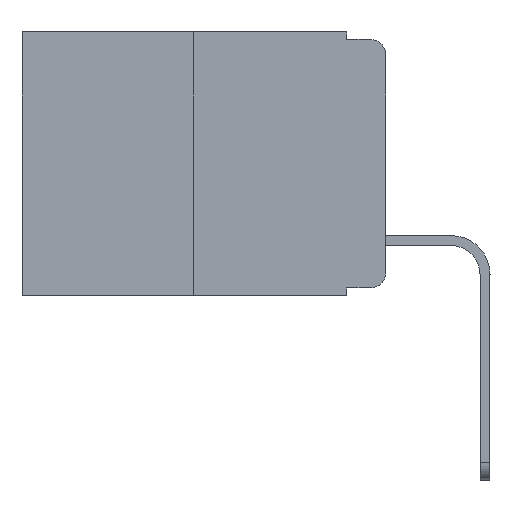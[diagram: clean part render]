
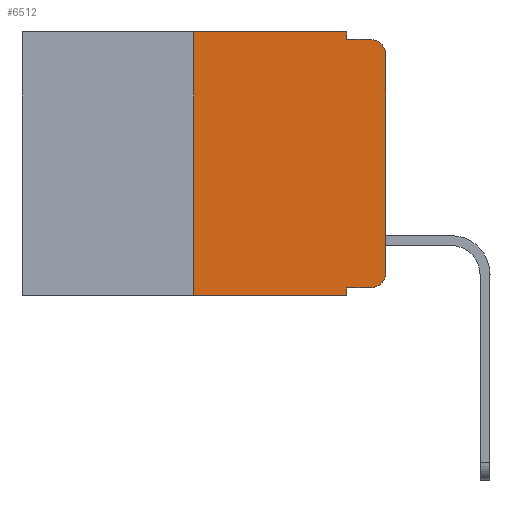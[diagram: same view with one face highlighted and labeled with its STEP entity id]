
A CAD part, left-side view. The second image highlights one B-rep face of the part: STEP entity #6512.
In plain terms, the highlighted planar face has unit normal (-1, 0, 0).
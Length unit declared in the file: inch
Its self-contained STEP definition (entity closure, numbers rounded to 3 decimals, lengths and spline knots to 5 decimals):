
#72 = CARTESIAN_POINT ( 'NONE',  ( 0., 0.051, -0.01 ) ) ;
#123 = CARTESIAN_POINT ( 'NONE',  ( 0., 0.051, 0. ) ) ;
#182 = CARTESIAN_POINT ( 'NONE',  ( 0., 0.25, 0. ) ) ;
#197 = EDGE_CURVE ( 'NONE', #8504, #10785, #8745, .T. ) ;
#387 = LINE ( 'NONE', #72, #3406 ) ;
#425 = VECTOR ( 'NONE', #4775, 39.37008 ) ;
#499 = EDGE_CURVE ( 'NONE', #6750, #7162, #10183, .T. ) ;
#504 = DIRECTION ( 'NONE',  ( 0., 0., -1. ) ) ;
#644 = PLANE ( 'NONE',  #7735 ) ;
#834 = VERTEX_POINT ( 'NONE', #10417 ) ;
#843 = CARTESIAN_POINT ( 'NONE',  ( 0., 0.051, 0. ) ) ;
#847 = ORIENTED_EDGE ( 'NONE', *, *, #5969, .T. ) ;
#1152 = ORIENTED_EDGE ( 'NONE', *, *, #8674, .F. ) ;
#1218 = ORIENTED_EDGE ( 'NONE', *, *, #499, .F. ) ;
#1422 = CARTESIAN_POINT ( 'NONE',  ( 0., 0.473, 0. ) ) ;
#1453 = VERTEX_POINT ( 'NONE', #5334 ) ;
#1470 = DIRECTION ( 'NONE',  ( 0., 0., -1. ) ) ;
#1519 = ORIENTED_EDGE ( 'NONE', *, *, #9599, .T. ) ;
#1961 = VECTOR ( 'NONE', #7259, 39.37008 ) ;
#2309 = DIRECTION ( 'NONE',  ( -1., 0., 0. ) ) ;
#2329 = CARTESIAN_POINT ( 'NONE',  ( 0., 0., -0.313 ) ) ;
#2451 = LINE ( 'NONE', #10314, #9060 ) ;
#2703 = CIRCLE ( 'NONE', #8658, 0.02 ) ;
#2772 = ORIENTED_EDGE ( 'NONE', *, *, #6137, .F. ) ;
#3129 = CARTESIAN_POINT ( 'NONE',  ( 0., 0.02, -0.313 ) ) ;
#3270 = DIRECTION ( 'NONE',  ( 0., 0., -1. ) ) ;
#3406 = VECTOR ( 'NONE', #5617, 39.37008 ) ;
#3453 = VERTEX_POINT ( 'NONE', #2329 ) ;
#3462 = CARTESIAN_POINT ( 'NONE',  ( 0., 0.051, -0.333 ) ) ;
#3577 = CARTESIAN_POINT ( 'NONE',  ( 0., 0.25, 0. ) ) ;
#3778 = EDGE_CURVE ( 'NONE', #834, #1453, #2451, .T. ) ;
#4098 = CARTESIAN_POINT ( 'NONE',  ( 0., 0.02, -0.03 ) ) ;
#4282 = EDGE_LOOP ( 'NONE', ( #847, #1519, #2772, #1152, #1218, #6490, #7884, #6775, #10735, #4455 ) ) ;
#4394 = VERTEX_POINT ( 'NONE', #7450 ) ;
#4455 = ORIENTED_EDGE ( 'NONE', *, *, #5741, .T. ) ;
#4775 = DIRECTION ( 'NONE',  ( 0., -1., 0. ) ) ;
#5334 = CARTESIAN_POINT ( 'NONE',  ( 0., 0.051, -0.343 ) ) ;
#5473 = DIRECTION ( 'NONE',  ( 0., 0., 1. ) ) ;
#5610 = AXIS2_PLACEMENT_3D ( 'NONE', #4098, #2309, #1470 ) ;
#5617 = DIRECTION ( 'NONE',  ( 0., -1., 0. ) ) ;
#5634 = VERTEX_POINT ( 'NONE', #9235 ) ;
#5646 = LINE ( 'NONE', #3577, #9093 ) ;
#5741 = EDGE_CURVE ( 'NONE', #10785, #3453, #2703, .T. ) ;
#5924 = CIRCLE ( 'NONE', #5610, 0.02 ) ;
#5969 = EDGE_CURVE ( 'NONE', #3453, #5634, #7565, .T. ) ;
#6130 = CARTESIAN_POINT ( 'NONE',  ( 0., 0.02, -0.333 ) ) ;
#6137 = EDGE_CURVE ( 'NONE', #4394, #8849, #387, .T. ) ;
#6301 = DIRECTION ( 'NONE',  ( 0., -1., 0. ) ) ;
#6380 = VECTOR ( 'NONE', #11082, 39.37008 ) ;
#6490 = ORIENTED_EDGE ( 'NONE', *, *, #8518, .F. ) ;
#6512 = ADVANCED_FACE ( 'NONE', ( #8415 ), #644, .F. ) ;
#6750 = VERTEX_POINT ( 'NONE', #182 ) ;
#6775 = ORIENTED_EDGE ( 'NONE', *, *, #7632, .F. ) ;
#7162 = VERTEX_POINT ( 'NONE', #843 ) ;
#7188 = DIRECTION ( 'NONE',  ( 0., 0., -1. ) ) ;
#7259 = DIRECTION ( 'NONE',  ( 0., 0., 1. ) ) ;
#7450 = CARTESIAN_POINT ( 'NONE',  ( 0., 0.051, -0.01 ) ) ;
#7565 = LINE ( 'NONE', #9949, #1961 ) ;
#7632 = EDGE_CURVE ( 'NONE', #8504, #1453, #8103, .T. ) ;
#7735 = AXIS2_PLACEMENT_3D ( 'NONE', #1422, #10728, #3270 ) ;
#7884 = ORIENTED_EDGE ( 'NONE', *, *, #3778, .T. ) ;
#7922 = LINE ( 'NONE', #123, #6380 ) ;
#8103 = LINE ( 'NONE', #11708, #8677 ) ;
#8382 = CARTESIAN_POINT ( 'NONE',  ( 0., 0.051, -0.333 ) ) ;
#8415 = FACE_OUTER_BOUND ( 'NONE', #4282, .T. ) ;
#8504 = VERTEX_POINT ( 'NONE', #3462 ) ;
#8511 = DIRECTION ( 'NONE',  ( 0., -1., 0. ) ) ;
#8518 = EDGE_CURVE ( 'NONE', #834, #6750, #5646, .T. ) ;
#8627 = CARTESIAN_POINT ( 'NONE',  ( 0., 0.02, -0.01 ) ) ;
#8658 = AXIS2_PLACEMENT_3D ( 'NONE', #3129, #10401, #504 ) ;
#8674 = EDGE_CURVE ( 'NONE', #7162, #4394, #7922, .T. ) ;
#8677 = VECTOR ( 'NONE', #7188, 39.37008 ) ;
#8745 = LINE ( 'NONE', #8382, #425 ) ;
#8849 = VERTEX_POINT ( 'NONE', #8627 ) ;
#9060 = VECTOR ( 'NONE', #8511, 39.37008 ) ;
#9093 = VECTOR ( 'NONE', #5473, 39.37008 ) ;
#9235 = CARTESIAN_POINT ( 'NONE',  ( 0., 0., -0.03 ) ) ;
#9599 = EDGE_CURVE ( 'NONE', #5634, #8849, #5924, .T. ) ;
#9949 = CARTESIAN_POINT ( 'NONE',  ( 0., 0., 0. ) ) ;
#10183 = LINE ( 'NONE', #11789, #11630 ) ;
#10314 = CARTESIAN_POINT ( 'NONE',  ( 0., 0.473, -0.343 ) ) ;
#10401 = DIRECTION ( 'NONE',  ( -1., 0., 0. ) ) ;
#10417 = CARTESIAN_POINT ( 'NONE',  ( 0., 0.25, -0.343 ) ) ;
#10728 = DIRECTION ( 'NONE',  ( 1., 0., 0. ) ) ;
#10735 = ORIENTED_EDGE ( 'NONE', *, *, #197, .T. ) ;
#10785 = VERTEX_POINT ( 'NONE', #6130 ) ;
#11082 = DIRECTION ( 'NONE',  ( 0., 0., -1. ) ) ;
#11630 = VECTOR ( 'NONE', #6301, 39.37008 ) ;
#11708 = CARTESIAN_POINT ( 'NONE',  ( 0., 0.051, 0. ) ) ;
#11789 = CARTESIAN_POINT ( 'NONE',  ( 0., 0.473, 0. ) ) ;
